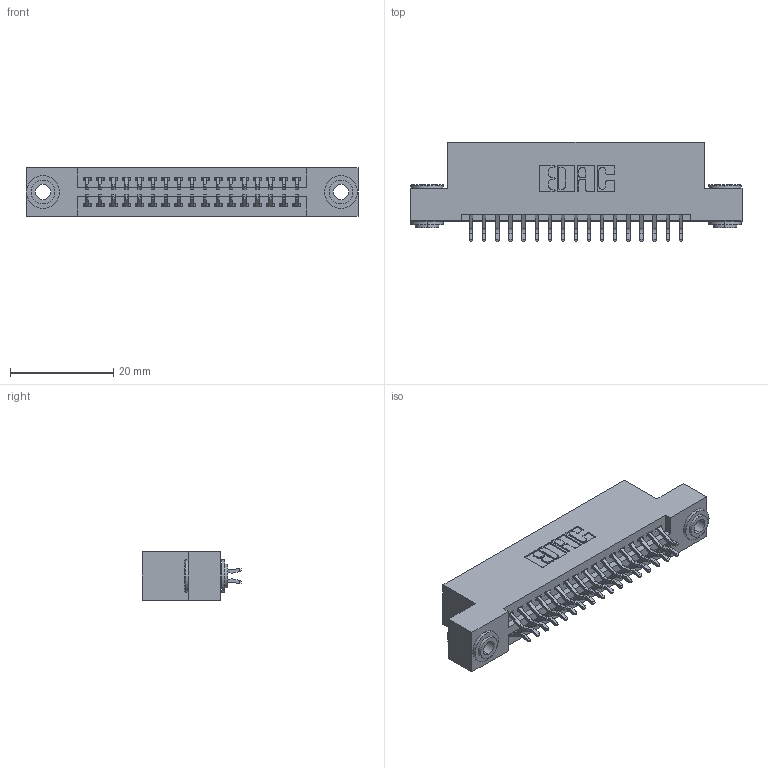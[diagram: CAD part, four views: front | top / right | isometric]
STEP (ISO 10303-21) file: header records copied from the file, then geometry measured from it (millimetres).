
FILE_DESCRIPTION (( 'STEP AP203' ), '1' );
FILE_NAME ('395-034-556-203.STEP', '2018-11-13T09:35:10', ( '' ), ( '' ), 'SwSTEP 2.0', 'SolidWorks 2016', '' );
FILE_SCHEMA (( 'CONFIG_CONTROL_DESIGN' ));
Length unit declared in the file: inch
Products named in the file (4): 345-250-002_345-250-002-102; 345 Part_Flush Mounting Lugs - 0.156 Dia-TH; 345-292-001_556 Tail; 395-034-556-203
Assembly tree (37 placements, depth 2):
  395-034-556-203
    345 Part_Flush Mounting Lugs - 0.156 Dia-TH
    345-292-001_556 Tail  x34
    345-250-002_345-250-002-102  x2
Bounding box: 64.39 x 19.24 x 9.4 mm (x, y, z)
Volume: 6040.8 mm3; surface area: 8620.3 mm2
Topology: 37 solids, 37 shells, 2068 faces, 6095 edges, 4014 vertices
Faces by surface type: plane 1348, cylinder 712, cone 8
Entity records: 17574 total; most frequent: CARTESIAN_POINT 2959, ORIENTED_EDGE 2874, DIRECTION 2659, EDGE_CURVE 1437, VECTOR 1205, LINE 1205, VERTEX_POINT 954, AXIS2_PLACEMENT_3D 727
